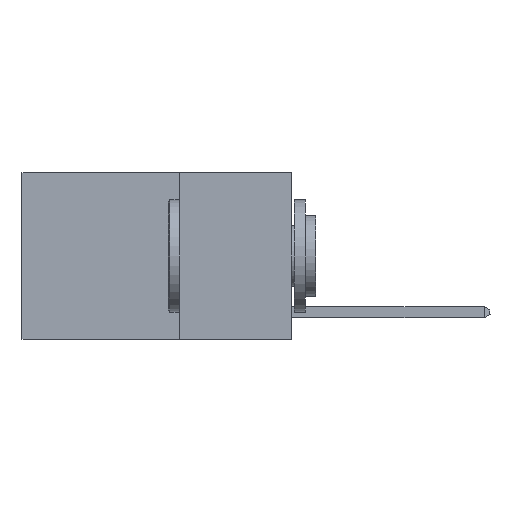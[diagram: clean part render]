
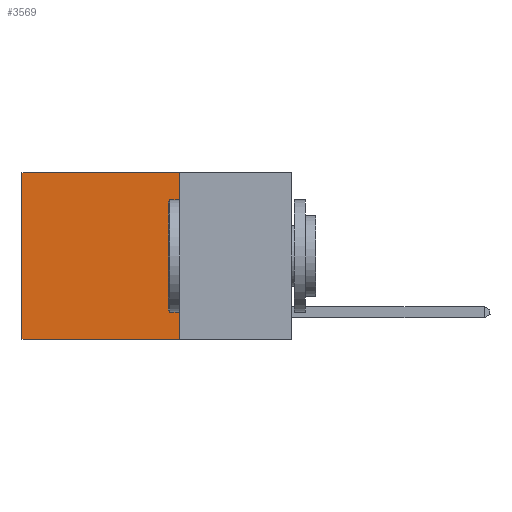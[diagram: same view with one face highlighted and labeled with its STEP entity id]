
A CAD part, left-side view. The second image highlights one B-rep face of the part: STEP entity #3569.
In plain terms, the highlighted planar face has unit normal (-1, 0, 0).
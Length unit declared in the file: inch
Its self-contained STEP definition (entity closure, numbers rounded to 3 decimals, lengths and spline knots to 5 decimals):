
#290 = DIRECTION ( 'NONE',  ( 0., 1., 0. ) ) ;
#292 = EDGE_CURVE ( 'NONE', #7994, #3805, #5427, .T. ) ;
#938 = DIRECTION ( 'NONE',  ( 0., 0., -1. ) ) ;
#1670 = CARTESIAN_POINT ( 'NONE',  ( 0.2625, 0.25, -0.37 ) ) ;
#1918 = DIRECTION ( 'NONE',  ( 0., 0., -1. ) ) ;
#2511 = VERTEX_POINT ( 'NONE', #7309 ) ;
#2550 = ORIENTED_EDGE ( 'NONE', *, *, #292, .F. ) ;
#2722 = CARTESIAN_POINT ( 'NONE',  ( 0.2625, 0.25, -0.37 ) ) ;
#2724 = VECTOR ( 'NONE', #8365, 39.37008 ) ;
#2814 = LINE ( 'NONE', #5949, #6354 ) ;
#2858 = EDGE_CURVE ( 'NONE', #3805, #2511, #8577, .T. ) ;
#2869 = CARTESIAN_POINT ( 'NONE',  ( 0.2625, 0.25, 0. ) ) ;
#3128 = AXIS2_PLACEMENT_3D ( 'NONE', #2869, #4281, #9212 ) ;
#3139 = CARTESIAN_POINT ( 'NONE',  ( 0.2625, 0.6, 0. ) ) ;
#3445 = CARTESIAN_POINT ( 'NONE',  ( 0.2625, 0.25, 0. ) ) ;
#3564 = PLANE ( 'NONE',  #3128 ) ;
#3569 = ADVANCED_FACE ( 'NONE', ( #8235 ), #3564, .F. ) ;
#3805 = VERTEX_POINT ( 'NONE', #1670 ) ;
#3814 = VERTEX_POINT ( 'NONE', #3139 ) ;
#4230 = CARTESIAN_POINT ( 'NONE',  ( 0.2625, 0.25, 0. ) ) ;
#4281 = DIRECTION ( 'NONE',  ( 1., 0., 0. ) ) ;
#5205 = VECTOR ( 'NONE', #1918, 39.37008 ) ;
#5332 = CARTESIAN_POINT ( 'NONE',  ( 0.2625, 0.25, 0. ) ) ;
#5427 = LINE ( 'NONE', #3445, #5205 ) ;
#5727 = EDGE_CURVE ( 'NONE', #7994, #3814, #8295, .T. ) ;
#5949 = CARTESIAN_POINT ( 'NONE',  ( 0.2625, 0.6, 0. ) ) ;
#6233 = EDGE_LOOP ( 'NONE', ( #6942, #7948, #2550, #7971 ) ) ;
#6354 = VECTOR ( 'NONE', #938, 39.37008 ) ;
#6431 = VECTOR ( 'NONE', #290, 39.37008 ) ;
#6942 = ORIENTED_EDGE ( 'NONE', *, *, #7582, .T. ) ;
#7309 = CARTESIAN_POINT ( 'NONE',  ( 0.2625, 0.6, -0.37 ) ) ;
#7582 = EDGE_CURVE ( 'NONE', #3814, #2511, #2814, .T. ) ;
#7948 = ORIENTED_EDGE ( 'NONE', *, *, #2858, .F. ) ;
#7971 = ORIENTED_EDGE ( 'NONE', *, *, #5727, .T. ) ;
#7994 = VERTEX_POINT ( 'NONE', #4230 ) ;
#8235 = FACE_OUTER_BOUND ( 'NONE', #6233, .T. ) ;
#8295 = LINE ( 'NONE', #5332, #6431 ) ;
#8365 = DIRECTION ( 'NONE',  ( 0., 1., 0. ) ) ;
#8577 = LINE ( 'NONE', #2722, #2724 ) ;
#9212 = DIRECTION ( 'NONE',  ( 0., 0., -1. ) ) ;
